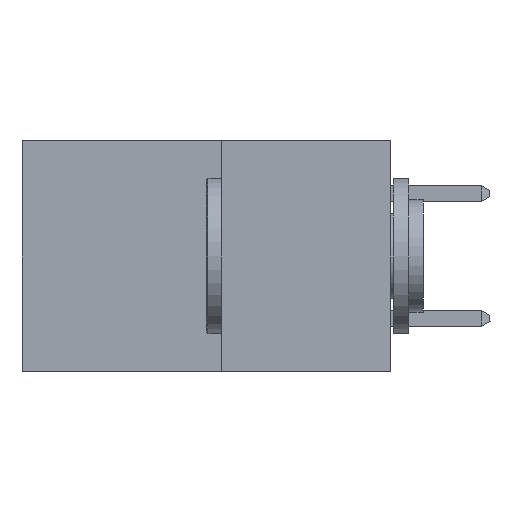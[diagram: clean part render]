
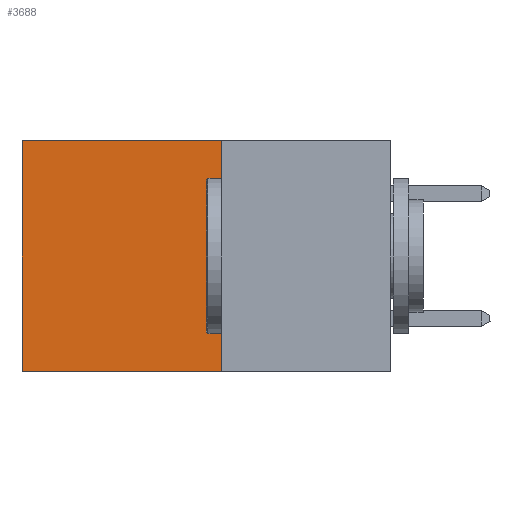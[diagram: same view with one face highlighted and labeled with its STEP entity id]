
A CAD part, left-side view. The second image highlights one B-rep face of the part: STEP entity #3688.
In plain terms, the highlighted planar face has unit normal (-1, 0, 0).
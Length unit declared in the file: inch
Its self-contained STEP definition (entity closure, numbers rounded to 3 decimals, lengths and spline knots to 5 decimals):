
#905 = LINE ( 'NONE', #9477, #5500 ) ;
#1019 = CARTESIAN_POINT ( 'NONE',  ( 0.277, 0.27, -0.37 ) ) ;
#3579 = ORIENTED_EDGE ( 'NONE', *, *, #19509, .F. ) ;
#3688 = ADVANCED_FACE ( 'NONE', ( #16326 ), #7679, .F. ) ;
#4112 = LINE ( 'NONE', #17355, #21087 ) ;
#4716 = CARTESIAN_POINT ( 'NONE',  ( 0.277, 0.59, -0.37 ) ) ;
#5500 = VECTOR ( 'NONE', #9243, 39.37008 ) ;
#5851 = LINE ( 'NONE', #16820, #9837 ) ;
#7269 = EDGE_CURVE ( 'NONE', #13406, #8572, #905, .T. ) ;
#7563 = DIRECTION ( 'NONE',  ( 0., 0., -1. ) ) ;
#7589 = DIRECTION ( 'NONE',  ( 1., 0., 0. ) ) ;
#7679 = PLANE ( 'NONE',  #20996 ) ;
#7724 = EDGE_CURVE ( 'NONE', #16157, #8572, #4112, .T. ) ;
#7736 = CARTESIAN_POINT ( 'NONE',  ( 0.277, 0.27, -0.37 ) ) ;
#8572 = VERTEX_POINT ( 'NONE', #4716 ) ;
#9243 = DIRECTION ( 'NONE',  ( 0., 1., 0. ) ) ;
#9477 = CARTESIAN_POINT ( 'NONE',  ( 0.277, 0.27, -0.37 ) ) ;
#9837 = VECTOR ( 'NONE', #21700, 39.37008 ) ;
#9871 = EDGE_LOOP ( 'NONE', ( #12831, #14812, #3579, #12925 ) ) ;
#9979 = VERTEX_POINT ( 'NONE', #13810 ) ;
#12166 = VECTOR ( 'NONE', #13317, 39.37008 ) ;
#12820 = EDGE_CURVE ( 'NONE', #9979, #16157, #16737, .T. ) ;
#12831 = ORIENTED_EDGE ( 'NONE', *, *, #7724, .T. ) ;
#12925 = ORIENTED_EDGE ( 'NONE', *, *, #12820, .T. ) ;
#13317 = DIRECTION ( 'NONE',  ( 0., 1., 0. ) ) ;
#13406 = VERTEX_POINT ( 'NONE', #1019 ) ;
#13810 = CARTESIAN_POINT ( 'NONE',  ( 0.277, 0.27, 0. ) ) ;
#14812 = ORIENTED_EDGE ( 'NONE', *, *, #7269, .F. ) ;
#16157 = VERTEX_POINT ( 'NONE', #18636 ) ;
#16326 = FACE_OUTER_BOUND ( 'NONE', #9871, .T. ) ;
#16702 = CARTESIAN_POINT ( 'NONE',  ( 0.277, 0.27, 0. ) ) ;
#16737 = LINE ( 'NONE', #16702, #12166 ) ;
#16820 = CARTESIAN_POINT ( 'NONE',  ( 0.277, 0.27, -0.37 ) ) ;
#17074 = DIRECTION ( 'NONE',  ( 0., 0., -1. ) ) ;
#17355 = CARTESIAN_POINT ( 'NONE',  ( 0.277, 0.59, -0.37 ) ) ;
#18636 = CARTESIAN_POINT ( 'NONE',  ( 0.277, 0.59, 0. ) ) ;
#19509 = EDGE_CURVE ( 'NONE', #9979, #13406, #5851, .T. ) ;
#20996 = AXIS2_PLACEMENT_3D ( 'NONE', #7736, #7589, #7563 ) ;
#21087 = VECTOR ( 'NONE', #17074, 39.37008 ) ;
#21700 = DIRECTION ( 'NONE',  ( 0., 0., -1. ) ) ;
